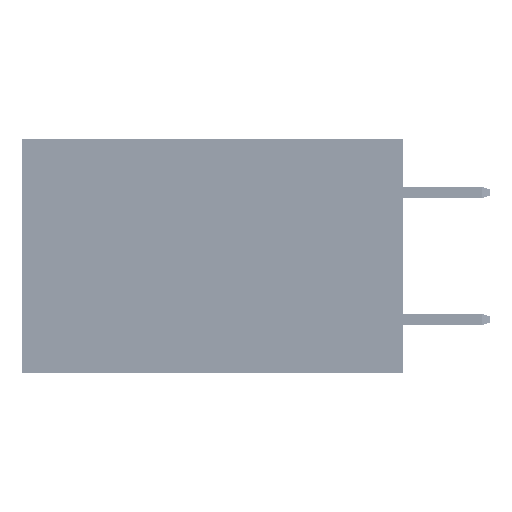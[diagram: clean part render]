
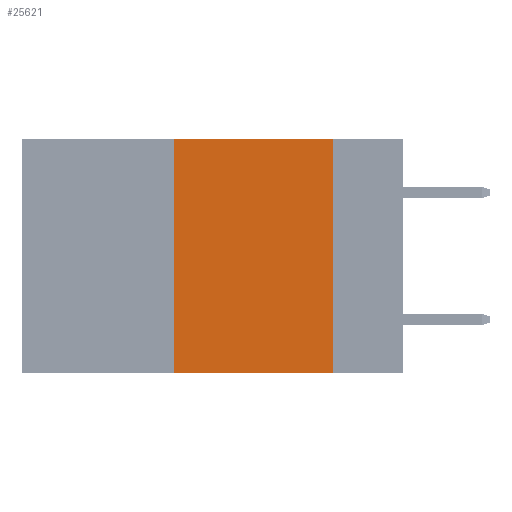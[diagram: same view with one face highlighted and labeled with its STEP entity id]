
A CAD part, left-side view. The second image highlights one B-rep face of the part: STEP entity #25621.
In plain terms, the highlighted planar face has unit normal (-1, 0, 0).
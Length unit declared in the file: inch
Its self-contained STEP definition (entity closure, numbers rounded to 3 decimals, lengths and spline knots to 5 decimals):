
#215 = PLANE ( 'NONE',  #6249 ) ;
#2899 = FACE_OUTER_BOUND ( 'NONE', #33789, .T. ) ;
#3655 = CARTESIAN_POINT ( 'NONE',  ( 0., 0.11, -0.37 ) ) ;
#3659 = VECTOR ( 'NONE', #19071, 39.37008 ) ;
#3695 = LINE ( 'NONE', #4641, #3659 ) ;
#4641 = CARTESIAN_POINT ( 'NONE',  ( 0., 0.6, 0. ) ) ;
#5988 = DIRECTION ( 'NONE',  ( 0., -1., 0. ) ) ;
#6249 = AXIS2_PLACEMENT_3D ( 'NONE', #10228, #47988, #36334 ) ;
#8160 = ORIENTED_EDGE ( 'NONE', *, *, #36091, .F. ) ;
#10085 = CARTESIAN_POINT ( 'NONE',  ( 0., 0.36, 0. ) ) ;
#10228 = CARTESIAN_POINT ( 'NONE',  ( 0., 0.6, 0. ) ) ;
#12351 = VECTOR ( 'NONE', #46554, 39.37008 ) ;
#13297 = VECTOR ( 'NONE', #5988, 39.37008 ) ;
#13417 = CARTESIAN_POINT ( 'NONE',  ( 0., 0.36, 0. ) ) ;
#14492 = CARTESIAN_POINT ( 'NONE',  ( 0., 0.11, 0. ) ) ;
#18185 = VERTEX_POINT ( 'NONE', #3655 ) ;
#18642 = DIRECTION ( 'NONE',  ( 0., 0., -1. ) ) ;
#19071 = DIRECTION ( 'NONE',  ( 0., -1., 0. ) ) ;
#24141 = VERTEX_POINT ( 'NONE', #10085 ) ;
#24149 = ORIENTED_EDGE ( 'NONE', *, *, #41833, .F. ) ;
#24969 = ORIENTED_EDGE ( 'NONE', *, *, #47290, .F. ) ;
#25621 = ADVANCED_FACE ( 'NONE', ( #2899 ), #215, .F. ) ;
#26601 = VERTEX_POINT ( 'NONE', #48058 ) ;
#27695 = EDGE_CURVE ( 'NONE', #26601, #18185, #31404, .T. ) ;
#31404 = LINE ( 'NONE', #39408, #13297 ) ;
#31738 = LINE ( 'NONE', #13417, #12351 ) ;
#33652 = VECTOR ( 'NONE', #18642, 39.37008 ) ;
#33789 = EDGE_LOOP ( 'NONE', ( #24969, #8160, #24149, #35593 ) ) ;
#35593 = ORIENTED_EDGE ( 'NONE', *, *, #27695, .T. ) ;
#36091 = EDGE_CURVE ( 'NONE', #24141, #43191, #3695, .T. ) ;
#36334 = DIRECTION ( 'NONE',  ( 0., 0., -1. ) ) ;
#39408 = CARTESIAN_POINT ( 'NONE',  ( 0., 0.6, -0.37 ) ) ;
#40817 = LINE ( 'NONE', #14492, #33652 ) ;
#41833 = EDGE_CURVE ( 'NONE', #26601, #24141, #31738, .T. ) ;
#43191 = VERTEX_POINT ( 'NONE', #46823 ) ;
#46554 = DIRECTION ( 'NONE',  ( 0., 0., 1. ) ) ;
#46823 = CARTESIAN_POINT ( 'NONE',  ( 0., 0.11, 0. ) ) ;
#47290 = EDGE_CURVE ( 'NONE', #43191, #18185, #40817, .T. ) ;
#47988 = DIRECTION ( 'NONE',  ( 1., 0., 0. ) ) ;
#48058 = CARTESIAN_POINT ( 'NONE',  ( 0., 0.36, -0.37 ) ) ;
